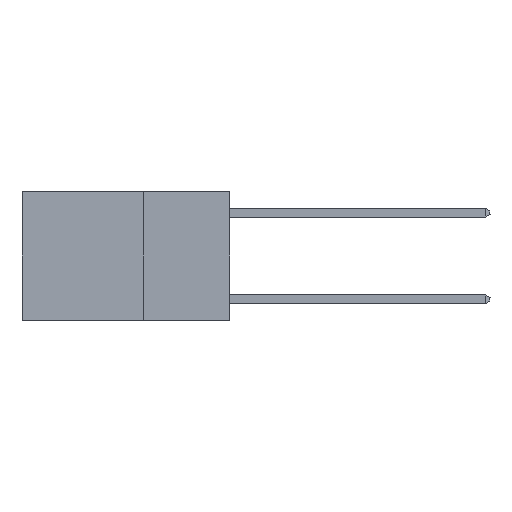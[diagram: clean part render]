
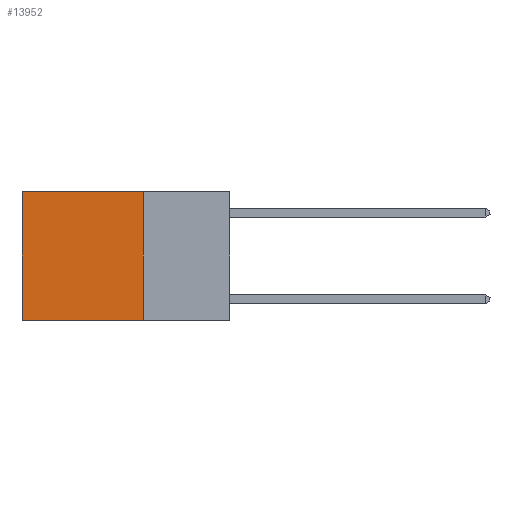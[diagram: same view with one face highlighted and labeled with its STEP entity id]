
A CAD part, left-side view. The second image highlights one B-rep face of the part: STEP entity #13952.
In plain terms, the highlighted planar face has unit normal (-1, 0, 0).
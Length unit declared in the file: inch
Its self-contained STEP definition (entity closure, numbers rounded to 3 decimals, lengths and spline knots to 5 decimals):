
#43 = LINE ( 'NONE', #4159, #9366 ) ;
#373 = VERTEX_POINT ( 'NONE', #15171 ) ;
#1404 = CARTESIAN_POINT ( 'NONE',  ( 0.2625, 0.6, -0.37 ) ) ;
#1450 = ORIENTED_EDGE ( 'NONE', *, *, #3369, .T. ) ;
#1772 = EDGE_CURVE ( 'NONE', #373, #16346, #11254, .T. ) ;
#2042 = EDGE_CURVE ( 'NONE', #14889, #16346, #12085, .T. ) ;
#2662 = PLANE ( 'NONE',  #6597 ) ;
#3018 = DIRECTION ( 'NONE',  ( 1., 0., 0. ) ) ;
#3023 = EDGE_CURVE ( 'NONE', #3910, #14889, #11258, .T. ) ;
#3369 = EDGE_CURVE ( 'NONE', #3910, #373, #43, .T. ) ;
#3445 = VECTOR ( 'NONE', #16558, 39.37008 ) ;
#3653 = ORIENTED_EDGE ( 'NONE', *, *, #1772, .T. ) ;
#3910 = VERTEX_POINT ( 'NONE', #13302 ) ;
#4097 = ORIENTED_EDGE ( 'NONE', *, *, #3023, .F. ) ;
#4159 = CARTESIAN_POINT ( 'NONE',  ( 0.2625, 0.25, 0. ) ) ;
#4235 = DIRECTION ( 'NONE',  ( 0., 0., -1. ) ) ;
#4851 = CARTESIAN_POINT ( 'NONE',  ( 0.2625, 0.25, 0. ) ) ;
#5540 = FACE_OUTER_BOUND ( 'NONE', #16335, .T. ) ;
#5633 = CARTESIAN_POINT ( 'NONE',  ( 0.2625, 0.25, -0.37 ) ) ;
#6597 = AXIS2_PLACEMENT_3D ( 'NONE', #6665, #3018, #4235 ) ;
#6665 = CARTESIAN_POINT ( 'NONE',  ( 0.2625, 0.25, 0. ) ) ;
#8020 = DIRECTION ( 'NONE',  ( 0., 1., 0. ) ) ;
#9366 = VECTOR ( 'NONE', #8020, 39.37008 ) ;
#10386 = ORIENTED_EDGE ( 'NONE', *, *, #2042, .F. ) ;
#10590 = VECTOR ( 'NONE', #15380, 39.37008 ) ;
#11084 = CARTESIAN_POINT ( 'NONE',  ( 0.2625, 0.25, -0.37 ) ) ;
#11254 = LINE ( 'NONE', #16556, #10590 ) ;
#11258 = LINE ( 'NONE', #4851, #3445 ) ;
#11983 = VECTOR ( 'NONE', #13573, 39.37008 ) ;
#12085 = LINE ( 'NONE', #5633, #11983 ) ;
#13302 = CARTESIAN_POINT ( 'NONE',  ( 0.2625, 0.25, 0. ) ) ;
#13573 = DIRECTION ( 'NONE',  ( 0., 1., 0. ) ) ;
#13952 = ADVANCED_FACE ( 'NONE', ( #5540 ), #2662, .F. ) ;
#14889 = VERTEX_POINT ( 'NONE', #11084 ) ;
#15171 = CARTESIAN_POINT ( 'NONE',  ( 0.2625, 0.6, 0. ) ) ;
#15380 = DIRECTION ( 'NONE',  ( 0., 0., -1. ) ) ;
#16335 = EDGE_LOOP ( 'NONE', ( #3653, #10386, #4097, #1450 ) ) ;
#16346 = VERTEX_POINT ( 'NONE', #1404 ) ;
#16556 = CARTESIAN_POINT ( 'NONE',  ( 0.2625, 0.6, 0. ) ) ;
#16558 = DIRECTION ( 'NONE',  ( 0., 0., -1. ) ) ;
